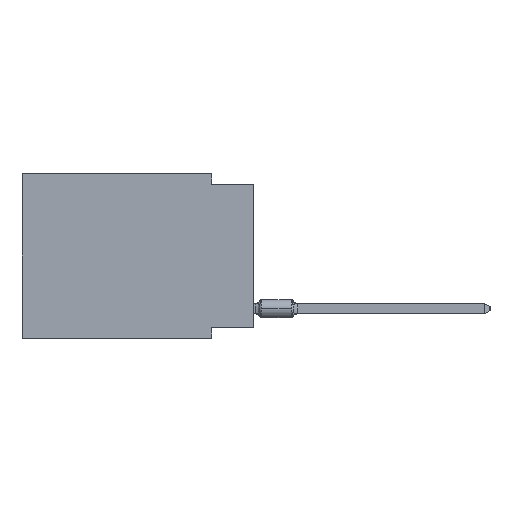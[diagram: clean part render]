
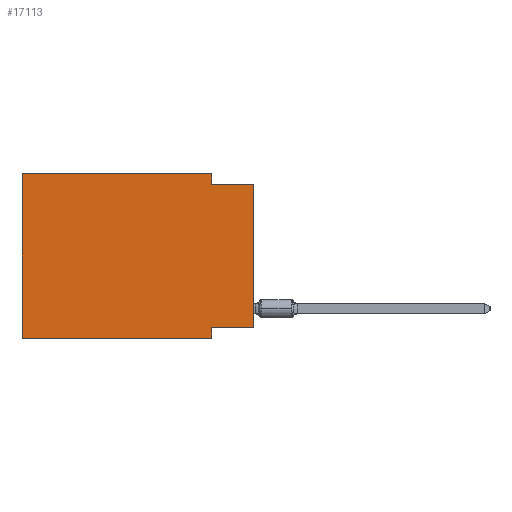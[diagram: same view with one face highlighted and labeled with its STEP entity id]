
A CAD part, left-side view. The second image highlights one B-rep face of the part: STEP entity #17113.
In plain terms, the highlighted planar face has unit normal (-1, 0, 0).
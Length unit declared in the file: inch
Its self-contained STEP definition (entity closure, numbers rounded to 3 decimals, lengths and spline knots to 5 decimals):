
#434 = LINE ( 'NONE', #3393, #40163 ) ;
#1216 = VERTEX_POINT ( 'NONE', #34352 ) ;
#1485 = CARTESIAN_POINT ( 'NONE',  ( 0., 0., 0. ) ) ;
#1726 = LINE ( 'NONE', #40439, #30433 ) ;
#1897 = LINE ( 'NONE', #1485, #1955 ) ;
#1955 = VECTOR ( 'NONE', #8019, 39.37008 ) ;
#3393 = CARTESIAN_POINT ( 'NONE',  ( 0., 0., -0.365 ) ) ;
#4484 = ORIENTED_EDGE ( 'NONE', *, *, #13954, .F. ) ;
#5266 = PLANE ( 'NONE',  #14548 ) ;
#8019 = DIRECTION ( 'NONE',  ( 0., 0., 1. ) ) ;
#8484 = LINE ( 'NONE', #40447, #12685 ) ;
#8564 = EDGE_CURVE ( 'NONE', #17569, #10275, #24620, .T. ) ;
#8634 = FACE_OUTER_BOUND ( 'NONE', #25444, .T. ) ;
#9278 = EDGE_CURVE ( 'NONE', #1216, #10716, #10247, .T. ) ;
#10247 = LINE ( 'NONE', #38636, #31843 ) ;
#10275 = VERTEX_POINT ( 'NONE', #28359 ) ;
#10716 = VERTEX_POINT ( 'NONE', #31246 ) ;
#11382 = CARTESIAN_POINT ( 'NONE',  ( 0., 0., -0.365 ) ) ;
#12099 = ORIENTED_EDGE ( 'NONE', *, *, #28303, .F. ) ;
#12685 = VECTOR ( 'NONE', #39606, 39.37008 ) ;
#13772 = EDGE_CURVE ( 'NONE', #17347, #1216, #35141, .T. ) ;
#13954 = EDGE_CURVE ( 'NONE', #17569, #17347, #30361, .T. ) ;
#14548 = AXIS2_PLACEMENT_3D ( 'NONE', #30904, #25035, #18295 ) ;
#14557 = DIRECTION ( 'NONE',  ( 0., -1., 0. ) ) ;
#15793 = CARTESIAN_POINT ( 'NONE',  ( 0., 0.55, -0.39 ) ) ;
#16545 = VECTOR ( 'NONE', #40041, 39.37008 ) ;
#17113 = ADVANCED_FACE ( 'NONE', ( #8634 ), #5266, .F. ) ;
#17347 = VERTEX_POINT ( 'NONE', #39904 ) ;
#17569 = VERTEX_POINT ( 'NONE', #15793 ) ;
#17850 = ORIENTED_EDGE ( 'NONE', *, *, #18993, .F. ) ;
#17884 = DIRECTION ( 'NONE',  ( 0., -1., 0. ) ) ;
#18295 = DIRECTION ( 'NONE',  ( 0., 0., -1. ) ) ;
#18624 = VERTEX_POINT ( 'NONE', #22616 ) ;
#18993 = EDGE_CURVE ( 'NONE', #21228, #35873, #434, .T. ) ;
#19286 = DIRECTION ( 'NONE',  ( 0., 0., -1. ) ) ;
#19770 = DIRECTION ( 'NONE',  ( 0., 1., 0. ) ) ;
#19820 = VECTOR ( 'NONE', #37888, 39.37008 ) ;
#20423 = CARTESIAN_POINT ( 'NONE',  ( 0., 0.55, -0.39 ) ) ;
#21228 = VERTEX_POINT ( 'NONE', #11382 ) ;
#22616 = CARTESIAN_POINT ( 'NONE',  ( 0., 0., -0.025 ) ) ;
#24620 = LINE ( 'NONE', #20423, #41191 ) ;
#25035 = DIRECTION ( 'NONE',  ( 1., 0., 0. ) ) ;
#25066 = CARTESIAN_POINT ( 'NONE',  ( 0., 0.55, 0. ) ) ;
#25174 = ORIENTED_EDGE ( 'NONE', *, *, #37924, .F. ) ;
#25444 = EDGE_LOOP ( 'NONE', ( #40719, #12099, #25642, #37588, #4484, #28223, #25174, #17850 ) ) ;
#25642 = ORIENTED_EDGE ( 'NONE', *, *, #9278, .F. ) ;
#27211 = CARTESIAN_POINT ( 'NONE',  ( 0., 0.55, 0. ) ) ;
#28223 = ORIENTED_EDGE ( 'NONE', *, *, #8564, .T. ) ;
#28303 = EDGE_CURVE ( 'NONE', #10716, #18624, #1726, .T. ) ;
#28359 = CARTESIAN_POINT ( 'NONE',  ( 0., 0.1, -0.39 ) ) ;
#30361 = LINE ( 'NONE', #27211, #16545 ) ;
#30433 = VECTOR ( 'NONE', #14557, 39.37008 ) ;
#30904 = CARTESIAN_POINT ( 'NONE',  ( 0., 0.55, 0. ) ) ;
#31246 = CARTESIAN_POINT ( 'NONE',  ( 0., 0.1, -0.025 ) ) ;
#31843 = VECTOR ( 'NONE', #19286, 39.37008 ) ;
#34352 = CARTESIAN_POINT ( 'NONE',  ( 0., 0.1, 0. ) ) ;
#35141 = LINE ( 'NONE', #25066, #19820 ) ;
#35873 = VERTEX_POINT ( 'NONE', #41364 ) ;
#37588 = ORIENTED_EDGE ( 'NONE', *, *, #13772, .F. ) ;
#37888 = DIRECTION ( 'NONE',  ( 0., -1., 0. ) ) ;
#37924 = EDGE_CURVE ( 'NONE', #35873, #10275, #8484, .T. ) ;
#38246 = EDGE_CURVE ( 'NONE', #21228, #18624, #1897, .T. ) ;
#38636 = CARTESIAN_POINT ( 'NONE',  ( 0., 0.1, 0. ) ) ;
#39606 = DIRECTION ( 'NONE',  ( 0., 0., -1. ) ) ;
#39904 = CARTESIAN_POINT ( 'NONE',  ( 0., 0.55, 0. ) ) ;
#40041 = DIRECTION ( 'NONE',  ( 0., 0., 1. ) ) ;
#40163 = VECTOR ( 'NONE', #19770, 39.37008 ) ;
#40439 = CARTESIAN_POINT ( 'NONE',  ( 0., 0., -0.025 ) ) ;
#40447 = CARTESIAN_POINT ( 'NONE',  ( 0., 0.1, -0.39 ) ) ;
#40719 = ORIENTED_EDGE ( 'NONE', *, *, #38246, .T. ) ;
#41191 = VECTOR ( 'NONE', #17884, 39.37008 ) ;
#41364 = CARTESIAN_POINT ( 'NONE',  ( 0., 0.1, -0.365 ) ) ;
